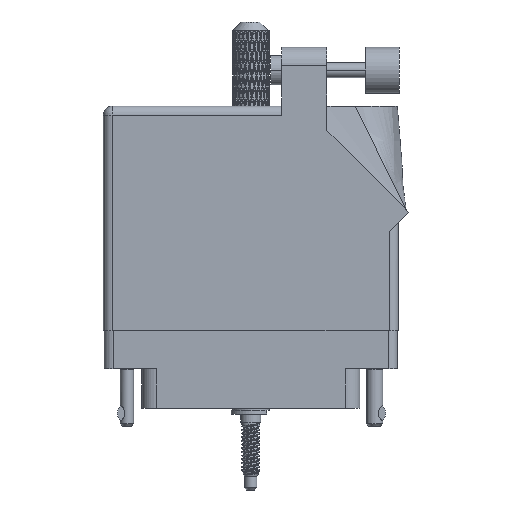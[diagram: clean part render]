
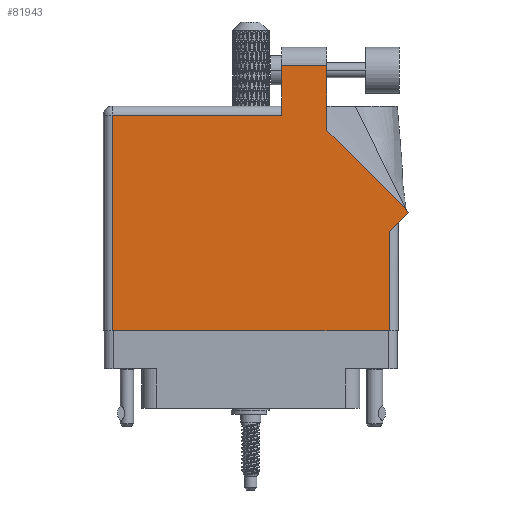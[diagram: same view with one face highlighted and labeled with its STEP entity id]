
A CAD part, front view. The second image highlights one B-rep face of the part: STEP entity #81943.
In plain terms, the highlighted face is planar.
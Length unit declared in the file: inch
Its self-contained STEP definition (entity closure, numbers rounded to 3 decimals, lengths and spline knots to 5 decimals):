
#102 = EDGE_CURVE ( 'NONE', #28167, #53996, #44453, .T. ) ;
#1297 = VECTOR ( 'NONE', #38741, 39.37008 ) ;
#1543 = ORIENTED_EDGE ( 'NONE', *, *, #61837, .T. ) ;
#2760 = CARTESIAN_POINT ( 'NONE',  ( 0.062, 1.468, 0. ) ) ;
#4184 = DIRECTION ( 'NONE',  ( -0.707, 0.707, 0. ) ) ;
#4787 = EDGE_CURVE ( 'NONE', #53996, #57904, #97679, .T. ) ;
#5593 = CARTESIAN_POINT ( 'NONE',  ( 1.217, 1.53, 0. ) ) ;
#8639 = EDGE_LOOP ( 'NONE', ( #105822, #87182, #13318, #61515, #47276, #98631, #1543, #69971, #95474 ) ) ;
#9825 = EDGE_CURVE ( 'NONE', #57904, #12954, #19873, .T. ) ;
#12165 = DIRECTION ( 'NONE',  ( 0., 1., 0. ) ) ;
#12825 = CARTESIAN_POINT ( 'NONE',  ( 2.01, 0.737, 0. ) ) ;
#12954 = VERTEX_POINT ( 'NONE', #105023 ) ;
#13318 = ORIENTED_EDGE ( 'NONE', *, *, #86298, .T. ) ;
#14716 = DIRECTION ( 'NONE',  ( 0.707, 0.707, 0. ) ) ;
#18118 = CARTESIAN_POINT ( 'NONE',  ( 1.524, 1.36442, 0. ) ) ;
#18214 = LINE ( 'NONE', #39418, #85724 ) ;
#18689 = CARTESIAN_POINT ( 'NONE',  ( 1.524, 1.805, 0. ) ) ;
#18870 = AXIS2_PLACEMENT_3D ( 'NONE', #54965, #28936, #48388 ) ;
#19873 = LINE ( 'NONE', #80239, #75006 ) ;
#21477 = LINE ( 'NONE', #74161, #76583 ) ;
#28167 = VERTEX_POINT ( 'NONE', #34681 ) ;
#28590 = VERTEX_POINT ( 'NONE', #97966 ) ;
#28936 = DIRECTION ( 'NONE',  ( 0., 0., -1. ) ) ;
#29990 = CARTESIAN_POINT ( 'NONE',  ( 1.217, 1.805, 0. ) ) ;
#33818 = CARTESIAN_POINT ( 'NONE',  ( 0.062, 0., 0. ) ) ;
#34681 = CARTESIAN_POINT ( 'NONE',  ( 1.217, 1.468, 0. ) ) ;
#34737 = VERTEX_POINT ( 'NONE', #65008 ) ;
#38741 = DIRECTION ( 'NONE',  ( -1., 0., 0. ) ) ;
#38956 = VECTOR ( 'NONE', #80367, 39.37008 ) ;
#39418 = CARTESIAN_POINT ( 'NONE',  ( 1.948, 0.737, 0. ) ) ;
#44453 = LINE ( 'NONE', #77386, #38956 ) ;
#46754 = VERTEX_POINT ( 'NONE', #18689 ) ;
#47276 = ORIENTED_EDGE ( 'NONE', *, *, #4787, .T. ) ;
#48034 = VECTOR ( 'NONE', #12165, 39.37008 ) ;
#48388 = DIRECTION ( 'NONE',  ( -1., 0., 0. ) ) ;
#50899 = VECTOR ( 'NONE', #85558, 39.37008 ) ;
#53996 = VERTEX_POINT ( 'NONE', #2760 ) ;
#54965 = CARTESIAN_POINT ( 'NONE',  ( 0., 1.53, 0. ) ) ;
#56360 = LINE ( 'NONE', #64825, #48034 ) ;
#57135 = DIRECTION ( 'NONE',  ( 0., 1., 0. ) ) ;
#57904 = VERTEX_POINT ( 'NONE', #33818 ) ;
#61515 = ORIENTED_EDGE ( 'NONE', *, *, #102, .T. ) ;
#61837 = EDGE_CURVE ( 'NONE', #12954, #66679, #18214, .T. ) ;
#62926 = DIRECTION ( 'NONE',  ( 1., 0., 0. ) ) ;
#63236 = LINE ( 'NONE', #12825, #81105 ) ;
#64825 = CARTESIAN_POINT ( 'NONE',  ( 1.524, 1.36442, 0. ) ) ;
#65008 = CARTESIAN_POINT ( 'NONE',  ( 2.08071, 0.80771, 0. ) ) ;
#66679 = VERTEX_POINT ( 'NONE', #109016 ) ;
#67965 = EDGE_CURVE ( 'NONE', #66679, #34737, #63236, .T. ) ;
#67995 = FACE_OUTER_BOUND ( 'NONE', #8639, .T. ) ;
#68530 = EDGE_CURVE ( 'NONE', #46754, #28590, #83792, .T. ) ;
#69971 = ORIENTED_EDGE ( 'NONE', *, *, #67965, .T. ) ;
#74161 = CARTESIAN_POINT ( 'NONE',  ( 2.08071, 0.80771, 0. ) ) ;
#75006 = VECTOR ( 'NONE', #62926, 39.37008 ) ;
#76583 = VECTOR ( 'NONE', #4184, 39.37008 ) ;
#77386 = CARTESIAN_POINT ( 'NONE',  ( 0., 1.468, 0. ) ) ;
#78917 = VERTEX_POINT ( 'NONE', #18118 ) ;
#79602 = EDGE_CURVE ( 'NONE', #34737, #78917, #21477, .T. ) ;
#80239 = CARTESIAN_POINT ( 'NONE',  ( 0., 0., 0. ) ) ;
#80367 = DIRECTION ( 'NONE',  ( -1., 0., 0. ) ) ;
#81105 = VECTOR ( 'NONE', #14716, 39.37008 ) ;
#81943 = ADVANCED_FACE ( 'NONE', ( #67995 ), #107649, .F. ) ;
#83792 = LINE ( 'NONE', #29990, #1297 ) ;
#85558 = DIRECTION ( 'NONE',  ( 0., -1., 0. ) ) ;
#85724 = VECTOR ( 'NONE', #57135, 39.37008 ) ;
#86298 = EDGE_CURVE ( 'NONE', #28590, #28167, #92787, .T. ) ;
#87182 = ORIENTED_EDGE ( 'NONE', *, *, #68530, .T. ) ;
#91316 = VECTOR ( 'NONE', #103164, 39.37008 ) ;
#92787 = LINE ( 'NONE', #5593, #91316 ) ;
#94760 = CARTESIAN_POINT ( 'NONE',  ( 0.062, 0., 0. ) ) ;
#95474 = ORIENTED_EDGE ( 'NONE', *, *, #79602, .T. ) ;
#97679 = LINE ( 'NONE', #94760, #50899 ) ;
#97966 = CARTESIAN_POINT ( 'NONE',  ( 1.217, 1.805, 0. ) ) ;
#98631 = ORIENTED_EDGE ( 'NONE', *, *, #9825, .T. ) ;
#99032 = EDGE_CURVE ( 'NONE', #78917, #46754, #56360, .T. ) ;
#103164 = DIRECTION ( 'NONE',  ( 0., -1., 0. ) ) ;
#105023 = CARTESIAN_POINT ( 'NONE',  ( 1.948, 0., 0. ) ) ;
#105822 = ORIENTED_EDGE ( 'NONE', *, *, #99032, .T. ) ;
#107649 = PLANE ( 'NONE',  #18870 ) ;
#109016 = CARTESIAN_POINT ( 'NONE',  ( 1.948, 0.675, 0. ) ) ;
